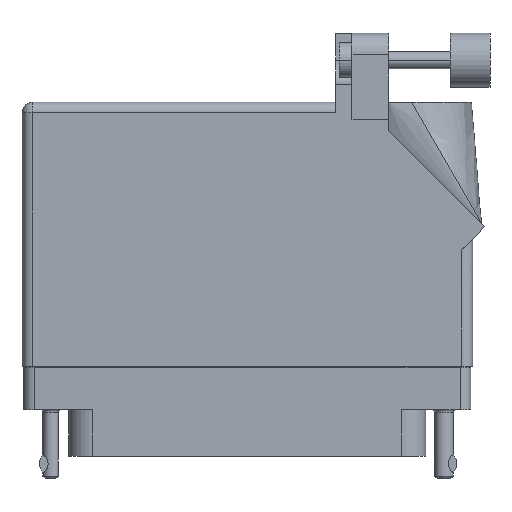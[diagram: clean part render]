
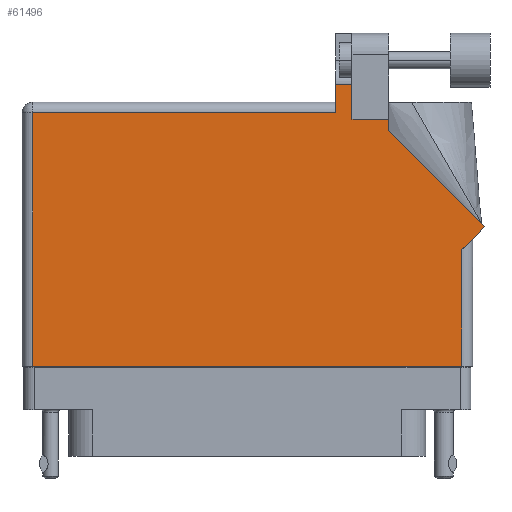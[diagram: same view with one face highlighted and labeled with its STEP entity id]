
A CAD part, front view. The second image highlights one B-rep face of the part: STEP entity #61496.
In plain terms, the highlighted face is planar.
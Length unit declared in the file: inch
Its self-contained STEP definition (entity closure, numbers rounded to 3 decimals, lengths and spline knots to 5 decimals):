
#2050 = CARTESIAN_POINT ( 'NONE',  ( 0.93777, 1.5315, 0.455 ) ) ;
#2214 = CARTESIAN_POINT ( 'NONE',  ( -1.306, 1.368, 0.455 ) ) ;
#3541 = EDGE_CURVE ( 'NONE', #5246, #7554, #32222, .T. ) ;
#3936 = VECTOR ( 'NONE', #52383, 39.37008 ) ;
#3983 = ORIENTED_EDGE ( 'NONE', *, *, #24365, .T. ) ;
#4005 = VECTOR ( 'NONE', #12932, 39.37008 ) ;
#4820 = VERTEX_POINT ( 'NONE', #59287 ) ;
#5246 = VERTEX_POINT ( 'NONE', #41324 ) ;
#5381 = VERTEX_POINT ( 'NONE', #41416 ) ;
#6518 = CARTESIAN_POINT ( 'NONE',  ( 0.607, 1.5315, 0.455 ) ) ;
#6803 = DIRECTION ( 'NONE',  ( 0., -1., 0. ) ) ;
#7002 = CARTESIAN_POINT ( 'NONE',  ( 1.37671, 0.70771, 0.455 ) ) ;
#7186 = CARTESIAN_POINT ( 'NONE',  ( 0.82, 1.33, 0.455 ) ) ;
#7554 = VERTEX_POINT ( 'NONE', #14091 ) ;
#7631 = CARTESIAN_POINT ( 'NONE',  ( -1.306, 1.43, 0.455 ) ) ;
#9457 = CARTESIAN_POINT ( 'NONE',  ( 1.306, 0.637, 0.455 ) ) ;
#9642 = VERTEX_POINT ( 'NONE', #49666 ) ;
#10481 = VECTOR ( 'NONE', #6803, 39.37008 ) ;
#11776 = CARTESIAN_POINT ( 'NONE',  ( 0.607, 1.33, 0.455 ) ) ;
#12526 = ORIENTED_EDGE ( 'NONE', *, *, #21610, .T. ) ;
#12719 = VERTEX_POINT ( 'NONE', #32461 ) ;
#12932 = DIRECTION ( 'NONE',  ( 1., 0., 0. ) ) ;
#14091 = CARTESIAN_POINT ( 'NONE',  ( 1.244, -0.1, 0.455 ) ) ;
#14240 = CARTESIAN_POINT ( 'NONE',  ( -1.244, 1.368, 0.455 ) ) ;
#14247 = LINE ( 'NONE', #15938, #10481 ) ;
#15524 = ORIENTED_EDGE ( 'NONE', *, *, #19134, .T. ) ;
#15938 = CARTESIAN_POINT ( 'NONE',  ( -1.244, -0.1, 0.455 ) ) ;
#16071 = ORIENTED_EDGE ( 'NONE', *, *, #20076, .T. ) ;
#16404 = CARTESIAN_POINT ( 'NONE',  ( 0.513, 1.5315, 0.455 ) ) ;
#16698 = ORIENTED_EDGE ( 'NONE', *, *, #33540, .T. ) ;
#17165 = DIRECTION ( 'NONE',  ( -1., 0., 0. ) ) ;
#17263 = LINE ( 'NONE', #9457, #24696 ) ;
#18108 = VERTEX_POINT ( 'NONE', #41579 ) ;
#19134 = EDGE_CURVE ( 'NONE', #27087, #4820, #32929, .T. ) ;
#19230 = CARTESIAN_POINT ( 'NONE',  ( 1.244, 0.637, 0.455 ) ) ;
#20076 = EDGE_CURVE ( 'NONE', #29401, #5246, #14247, .T. ) ;
#20360 = ORIENTED_EDGE ( 'NONE', *, *, #33612, .T. ) ;
#20478 = LINE ( 'NONE', #7186, #25726 ) ;
#21065 = VECTOR ( 'NONE', #45635, 39.37008 ) ;
#21373 = ORIENTED_EDGE ( 'NONE', *, *, #47918, .T. ) ;
#21610 = EDGE_CURVE ( 'NONE', #7554, #5381, #33639, .T. ) ;
#21726 = VECTOR ( 'NONE', #26364, 39.37008 ) ;
#21785 = LINE ( 'NONE', #40856, #21726 ) ;
#22095 = LINE ( 'NONE', #2214, #60569 ) ;
#23812 = VERTEX_POINT ( 'NONE', #26644 ) ;
#24365 = EDGE_CURVE ( 'NONE', #18108, #23812, #21785, .T. ) ;
#24696 = VECTOR ( 'NONE', #28581, 39.37008 ) ;
#25726 = VECTOR ( 'NONE', #45166, 39.37008 ) ;
#26364 = DIRECTION ( 'NONE',  ( 0., 1., 0. ) ) ;
#26644 = CARTESIAN_POINT ( 'NONE',  ( 0.82, 1.33, 0.455 ) ) ;
#27087 = VERTEX_POINT ( 'NONE', #16404 ) ;
#27253 = LINE ( 'NONE', #7002, #28764 ) ;
#28581 = DIRECTION ( 'NONE',  ( 0.707, 0.707, 0. ) ) ;
#28764 = VECTOR ( 'NONE', #44956, 39.37008 ) ;
#29401 = VERTEX_POINT ( 'NONE', #14240 ) ;
#30690 = EDGE_CURVE ( 'NONE', #5381, #12719, #17263, .T. ) ;
#31125 = DIRECTION ( 'NONE',  ( -1., 0., 0. ) ) ;
#31138 = DIRECTION ( 'NONE',  ( -1., 0., 0. ) ) ;
#32214 = VECTOR ( 'NONE', #42031, 39.37008 ) ;
#32222 = LINE ( 'NONE', #60160, #4005 ) ;
#32461 = CARTESIAN_POINT ( 'NONE',  ( 1.37671, 0.70771, 0.455 ) ) ;
#32510 = CARTESIAN_POINT ( 'NONE',  ( 0.513, 1.43, 0.455 ) ) ;
#32929 = LINE ( 'NONE', #32510, #32214 ) ;
#33540 = EDGE_CURVE ( 'NONE', #4820, #29401, #22095, .T. ) ;
#33612 = EDGE_CURVE ( 'NONE', #12719, #18108, #27253, .T. ) ;
#33639 = LINE ( 'NONE', #19230, #3936 ) ;
#35046 = ORIENTED_EDGE ( 'NONE', *, *, #30690, .T. ) ;
#35307 = LINE ( 'NONE', #2050, #47988 ) ;
#39090 = ORIENTED_EDGE ( 'NONE', *, *, #47594, .T. ) ;
#40856 = CARTESIAN_POINT ( 'NONE',  ( 0.82, 1.26442, 0.455 ) ) ;
#40918 = VERTEX_POINT ( 'NONE', #6518 ) ;
#41324 = CARTESIAN_POINT ( 'NONE',  ( -1.244, -0.1, 0.455 ) ) ;
#41416 = CARTESIAN_POINT ( 'NONE',  ( 1.244, 0.575, 0.455 ) ) ;
#41579 = CARTESIAN_POINT ( 'NONE',  ( 0.82, 1.26442, 0.455 ) ) ;
#42031 = DIRECTION ( 'NONE',  ( 0., -1., 0. ) ) ;
#42833 = ORIENTED_EDGE ( 'NONE', *, *, #3541, .T. ) ;
#43890 = AXIS2_PLACEMENT_3D ( 'NONE', #7631, #54702, #31125 ) ;
#44783 = PLANE ( 'NONE',  #43890 ) ;
#44956 = DIRECTION ( 'NONE',  ( -0.707, 0.707, 0. ) ) ;
#45166 = DIRECTION ( 'NONE',  ( -1., 0., 0. ) ) ;
#45635 = DIRECTION ( 'NONE',  ( 0., 1., 0. ) ) ;
#47594 = EDGE_CURVE ( 'NONE', #40918, #27087, #35307, .T. ) ;
#47918 = EDGE_CURVE ( 'NONE', #23812, #9642, #20478, .T. ) ;
#47988 = VECTOR ( 'NONE', #31138, 39.37008 ) ;
#49666 = CARTESIAN_POINT ( 'NONE',  ( 0.607, 1.33, 0.455 ) ) ;
#50700 = FACE_OUTER_BOUND ( 'NONE', #56891, .T. ) ;
#51441 = LINE ( 'NONE', #11776, #21065 ) ;
#52383 = DIRECTION ( 'NONE',  ( 0., 1., 0. ) ) ;
#54702 = DIRECTION ( 'NONE',  ( 0., 0., -1. ) ) ;
#56891 = EDGE_LOOP ( 'NONE', ( #57482, #39090, #15524, #16698, #16071, #42833, #12526, #35046, #20360, #3983, #21373 ) ) ;
#57482 = ORIENTED_EDGE ( 'NONE', *, *, #58686, .T. ) ;
#58686 = EDGE_CURVE ( 'NONE', #9642, #40918, #51441, .T. ) ;
#59287 = CARTESIAN_POINT ( 'NONE',  ( 0.513, 1.368, 0.455 ) ) ;
#60160 = CARTESIAN_POINT ( 'NONE',  ( -1.306, -0.1, 0.455 ) ) ;
#60569 = VECTOR ( 'NONE', #17165, 39.37008 ) ;
#61496 = ADVANCED_FACE ( 'NONE', ( #50700 ), #44783, .F. ) ;
